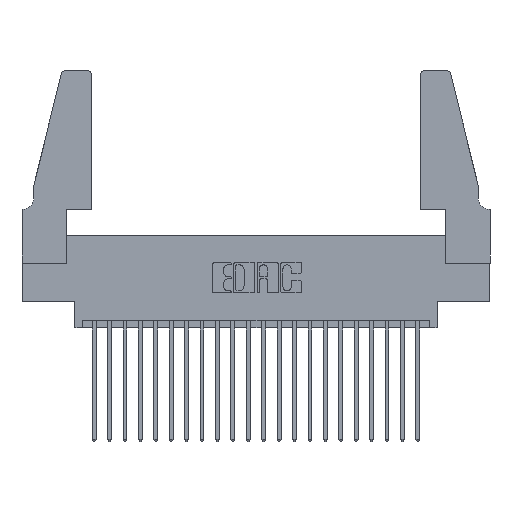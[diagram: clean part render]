
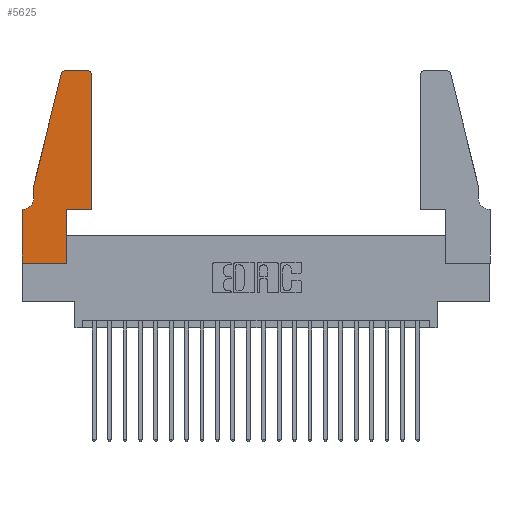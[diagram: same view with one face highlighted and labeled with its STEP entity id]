
A CAD part, top view. The second image highlights one B-rep face of the part: STEP entity #5625.
In plain terms, the highlighted planar face has unit normal (0, 0, 1).
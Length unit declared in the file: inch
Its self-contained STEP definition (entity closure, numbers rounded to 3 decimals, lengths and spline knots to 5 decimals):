
#76 = EDGE_CURVE ( 'NONE', #1844, #19083, #22153, .T. ) ;
#88 = ORIENTED_EDGE ( 'NONE', *, *, #20828, .T. ) ;
#165 = ORIENTED_EDGE ( 'NONE', *, *, #76, .T. ) ;
#1325 = AXIS2_PLACEMENT_3D ( 'NONE', #3769, #15895, #5568 ) ;
#1585 = DIRECTION ( 'NONE',  ( -0.239, -0.971, 0. ) ) ;
#1833 = CARTESIAN_POINT ( 'NONE',  ( 0.4505, 0.35, 0.37 ) ) ;
#1844 = VERTEX_POINT ( 'NONE', #15699 ) ;
#2043 = ORIENTED_EDGE ( 'NONE', *, *, #16577, .T. ) ;
#2306 = CARTESIAN_POINT ( 'NONE',  ( 0.4505, 0.35, 0.37 ) ) ;
#2550 = ORIENTED_EDGE ( 'NONE', *, *, #10543, .T. ) ;
#3133 = CARTESIAN_POINT ( 'NONE',  ( 0.0755, 0.42, 0.37 ) ) ;
#3200 = DIRECTION ( 'NONE',  ( 0., 0., 1. ) ) ;
#3505 = LINE ( 'NONE', #11194, #16779 ) ;
#3664 = DIRECTION ( 'NONE',  ( 1., 0., 0. ) ) ;
#3698 = ORIENTED_EDGE ( 'NONE', *, *, #15175, .T. ) ;
#3769 = CARTESIAN_POINT ( 'NONE',  ( 0.0055, 0.42, 0.37 ) ) ;
#3831 = ORIENTED_EDGE ( 'NONE', *, *, #3856, .T. ) ;
#3856 = EDGE_CURVE ( 'NONE', #21084, #4471, #21226, .T. ) ;
#3869 = VERTEX_POINT ( 'NONE', #20958 ) ;
#3964 = EDGE_CURVE ( 'NONE', #16365, #7606, #19179, .T. ) ;
#4471 = VERTEX_POINT ( 'NONE', #19080 ) ;
#4480 = DIRECTION ( 'NONE',  ( 0., 0., 1. ) ) ;
#4533 = EDGE_CURVE ( 'NONE', #19083, #18289, #17605, .T. ) ;
#4568 = ORIENTED_EDGE ( 'NONE', *, *, #20697, .T. ) ;
#5459 = VECTOR ( 'NONE', #8086, 39.37008 ) ;
#5482 = CARTESIAN_POINT ( 'NONE',  ( 0.284, 1.22, 0.37 ) ) ;
#5559 = VECTOR ( 'NONE', #5899, 39.37008 ) ;
#5568 = DIRECTION ( 'NONE',  ( -1., 0., 0. ) ) ;
#5625 = ADVANCED_FACE ( 'NONE', ( #14971 ), #14888, .T. ) ;
#5662 = LINE ( 'NONE', #17211, #14357 ) ;
#5899 = DIRECTION ( 'NONE',  ( 0., 1., 0. ) ) ;
#5996 = ORIENTED_EDGE ( 'NONE', *, *, #15011, .T. ) ;
#6310 = CARTESIAN_POINT ( 'NONE',  ( 0.0755, 0.35, 0.37 ) ) ;
#6800 = CARTESIAN_POINT ( 'NONE',  ( 0., 0., 0.37 ) ) ;
#7007 = CARTESIAN_POINT ( 'NONE',  ( 0., 0.35, 0.37 ) ) ;
#7109 = EDGE_CURVE ( 'NONE', #8879, #1844, #19563, .T. ) ;
#7249 = DIRECTION ( 'NONE',  ( 1., 0., 0. ) ) ;
#7606 = VERTEX_POINT ( 'NONE', #16785 ) ;
#7785 = DIRECTION ( 'NONE',  ( 0., -1., 0. ) ) ;
#7860 = ORIENTED_EDGE ( 'NONE', *, *, #20542, .T. ) ;
#7956 = CARTESIAN_POINT ( 'NONE',  ( 0., 0.35, 0.37 ) ) ;
#8086 = DIRECTION ( 'NONE',  ( -1., 0., 0. ) ) ;
#8369 = VECTOR ( 'NONE', #3664, 39.37008 ) ;
#8525 = CIRCLE ( 'NONE', #20709, 0.03 ) ;
#8740 = CARTESIAN_POINT ( 'NONE',  ( 0.4505, 0.35, 0.37 ) ) ;
#8879 = VERTEX_POINT ( 'NONE', #9916 ) ;
#9075 = ORIENTED_EDGE ( 'NONE', *, *, #7109, .T. ) ;
#9419 = DIRECTION ( 'NONE',  ( 0., 1., 0. ) ) ;
#9799 = ORIENTED_EDGE ( 'NONE', *, *, #3964, .T. ) ;
#9916 = CARTESIAN_POINT ( 'NONE',  ( 0.25487, 1.22718, 0.37 ) ) ;
#10543 = EDGE_CURVE ( 'NONE', #16896, #20368, #5662, .T. ) ;
#11099 = VECTOR ( 'NONE', #17767, 39.37008 ) ;
#11194 = CARTESIAN_POINT ( 'NONE',  ( 0.2865, 0.35, 0.37 ) ) ;
#12402 = VERTEX_POINT ( 'NONE', #13997 ) ;
#12457 = VECTOR ( 'NONE', #15995, 39.37008 ) ;
#13343 = AXIS2_PLACEMENT_3D ( 'NONE', #7956, #4480, #16550 ) ;
#13712 = CARTESIAN_POINT ( 'NONE',  ( 0.4205, 1.22, 0.37 ) ) ;
#13997 = CARTESIAN_POINT ( 'NONE',  ( 0.2865, 0., 0.37 ) ) ;
#14006 = AXIS2_PLACEMENT_3D ( 'NONE', #13712, #3200, #15371 ) ;
#14332 = CARTESIAN_POINT ( 'NONE',  ( 0.2605, 1.25, 0.37 ) ) ;
#14357 = VECTOR ( 'NONE', #18868, 39.37008 ) ;
#14638 = VECTOR ( 'NONE', #1585, 39.37008 ) ;
#14888 = PLANE ( 'NONE',  #13343 ) ;
#14971 = FACE_OUTER_BOUND ( 'NONE', #17846, .T. ) ;
#15011 = EDGE_CURVE ( 'NONE', #7606, #21084, #21520, .T. ) ;
#15175 = EDGE_CURVE ( 'NONE', #3869, #16365, #21772, .T. ) ;
#15371 = DIRECTION ( 'NONE',  ( 1., 0., 0. ) ) ;
#15553 = LINE ( 'NONE', #19364, #11099 ) ;
#15699 = CARTESIAN_POINT ( 'NONE',  ( 0.0755, 0.5, 0.37 ) ) ;
#15895 = DIRECTION ( 'NONE',  ( 0., 0., -1. ) ) ;
#15995 = DIRECTION ( 'NONE',  ( -1., 0., 0. ) ) ;
#16365 = VERTEX_POINT ( 'NONE', #8740 ) ;
#16550 = DIRECTION ( 'NONE',  ( 1., 0., 0. ) ) ;
#16577 = EDGE_CURVE ( 'NONE', #20368, #12402, #15553, .T. ) ;
#16773 = ORIENTED_EDGE ( 'NONE', *, *, #4533, .T. ) ;
#16779 = VECTOR ( 'NONE', #9419, 39.37008 ) ;
#16785 = CARTESIAN_POINT ( 'NONE',  ( 0.4505, 1.22, 0.37 ) ) ;
#16896 = VERTEX_POINT ( 'NONE', #7007 ) ;
#17211 = CARTESIAN_POINT ( 'NONE',  ( 0., 0., 0.37 ) ) ;
#17239 = CARTESIAN_POINT ( 'NONE',  ( 0.4205, 1.25, 0.37 ) ) ;
#17484 = DIRECTION ( 'NONE',  ( 0., 0., 1. ) ) ;
#17605 = CIRCLE ( 'NONE', #1325, 0.07 ) ;
#17767 = DIRECTION ( 'NONE',  ( 1., 0., 0. ) ) ;
#17846 = EDGE_LOOP ( 'NONE', ( #3831, #7860, #9075, #165, #16773, #88, #2550, #2043, #4568, #3698, #9799, #5996 ) ) ;
#18289 = VERTEX_POINT ( 'NONE', #21595 ) ;
#18868 = DIRECTION ( 'NONE',  ( 0., -1., 0. ) ) ;
#19080 = CARTESIAN_POINT ( 'NONE',  ( 0.284, 1.25, 0.37 ) ) ;
#19083 = VERTEX_POINT ( 'NONE', #3133 ) ;
#19090 = LINE ( 'NONE', #6310, #5459 ) ;
#19179 = LINE ( 'NONE', #2306, #5559 ) ;
#19364 = CARTESIAN_POINT ( 'NONE',  ( 0., 0., 0.37 ) ) ;
#19563 = LINE ( 'NONE', #22115, #14638 ) ;
#20368 = VERTEX_POINT ( 'NONE', #6800 ) ;
#20542 = EDGE_CURVE ( 'NONE', #4471, #8879, #8525, .T. ) ;
#20697 = EDGE_CURVE ( 'NONE', #12402, #3869, #3505, .T. ) ;
#20709 = AXIS2_PLACEMENT_3D ( 'NONE', #5482, #17484, #7249 ) ;
#20828 = EDGE_CURVE ( 'NONE', #18289, #16896, #19090, .T. ) ;
#20938 = CARTESIAN_POINT ( 'NONE',  ( 0.0755, 0.5, 0.37 ) ) ;
#20958 = CARTESIAN_POINT ( 'NONE',  ( 0.2865, 0.35, 0.37 ) ) ;
#21084 = VERTEX_POINT ( 'NONE', #17239 ) ;
#21226 = LINE ( 'NONE', #14332, #12457 ) ;
#21520 = CIRCLE ( 'NONE', #14006, 0.03 ) ;
#21595 = CARTESIAN_POINT ( 'NONE',  ( 0.0055, 0.35, 0.37 ) ) ;
#21630 = VECTOR ( 'NONE', #7785, 39.37008 ) ;
#21772 = LINE ( 'NONE', #1833, #8369 ) ;
#22115 = CARTESIAN_POINT ( 'NONE',  ( 0.0755, 0.5, 0.37 ) ) ;
#22153 = LINE ( 'NONE', #20938, #21630 ) ;
